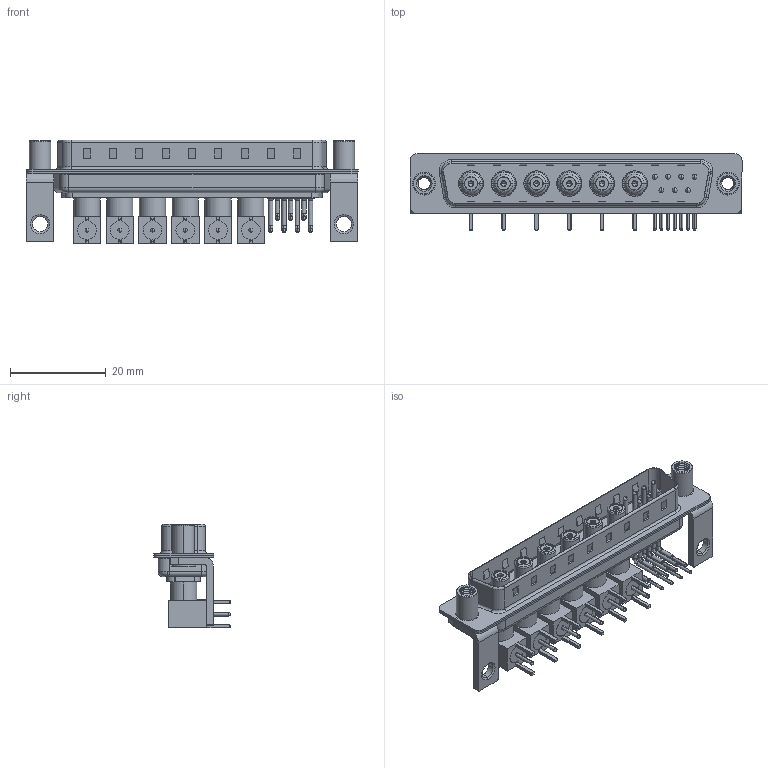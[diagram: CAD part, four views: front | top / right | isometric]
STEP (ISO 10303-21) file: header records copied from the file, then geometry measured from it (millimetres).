
FILE_DESCRIPTION (( 'STEP AP203' ), '1' );
FILE_NAME ('629-13W6640-7T6.STEP', '2022-05-14T19:23:55', ( '' ), ( '' ), 'SwSTEP 2.0', 'SolidWorks 2020', '' );
FILE_SCHEMA (( 'CONFIG_CONTROL_DESIGN' ));
Length unit declared in the file: millimetre
Products named in the file (21): Insulator RA Pin; 629Combo Stabilizer Bracket; Co-Ax Jack Assy_RA; 629-13W6640-7T6; Socket_RA; Co-Ax Jack_RA PC Tail; 629Combo Shell Rear_37 Contacts; 629Combo Threaded Standoff_D; 629Combo Contact Row 2; Insulator Socket 2; 629Combo Shell Front_37 Contacts; 629Combo Contact Row 1; Insulator Socket; 629Combo Housing_13W6; Locking Collar; RA Back Shell
Assembly tree (62 placements, depth 3):
  629-13W6640-7T6
    629Combo Housing_13W6
    629Combo Shell Rear_37 Contacts
    629Combo Shell Front_37 Contacts
    629Combo Stabilizer Bracket  x2
    629Combo Threaded Standoff_D  x2
    Co-Ax Jack Assy_RA
      Co-Ax Jack_RA PC Tail
      Insulator Socket
      Insulator Socket 2
      Locking Collar
      Socket_RA
      RA Back Shell
      Insulator RA Pin
    Co-Ax Jack Assy_RA
      Co-Ax Jack_RA PC Tail
      Insulator Socket
      Insulator Socket 2
      Locking Collar
      Socket_RA
      RA Back Shell
      Insulator RA Pin
    Co-Ax Jack Assy_RA
      Co-Ax Jack_RA PC Tail
      Insulator Socket
      Insulator Socket 2
      Locking Collar
      Socket_RA
      RA Back Shell
      Insulator RA Pin
    Co-Ax Jack Assy_RA
      Co-Ax Jack_RA PC Tail
      Insulator Socket
      Insulator Socket 2
      Locking Collar
      Socket_RA
      RA Back Shell
      Insulator RA Pin
    Co-Ax Jack Assy_RA
      Co-Ax Jack_RA PC Tail
      Insulator Socket
      Insulator Socket 2
      Locking Collar
      Socket_RA
      RA Back Shell
      Insulator RA Pin
    Co-Ax Jack Assy_RA
      Co-Ax Jack_RA PC Tail
      Insulator Socket
      Insulator Socket 2
      Locking Collar
      Socket_RA
      RA Back Shell
      Insulator RA Pin
    629Combo Contact Row 1  x4
    629Combo Contact Row 2  x3
Bounding box: 69.4 x 16 x 21.71 mm (x, y, z)
Volume: 5920.8 mm3; surface area: 15875.3 mm2
Topology: 56 solids, 56 shells, 2192 faces, 5575 edges, 3544 vertices
Faces by surface type: plane 1015, cylinder 867, cone 158, torus 86, bspline 54, sphere 12
Entity records: 32372 total; most frequent: CARTESIAN_POINT 7331, DIRECTION 4702, ORIENTED_EDGE 4416, EDGE_CURVE 2208, AXIS2_PLACEMENT_3D 1682, VERTEX_POINT 1420, LINE 1338, VECTOR 1338
